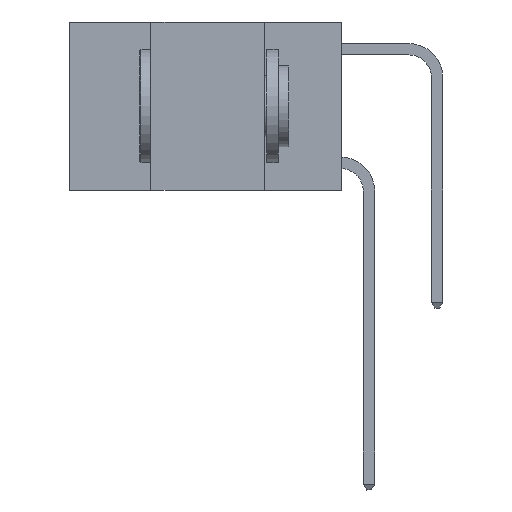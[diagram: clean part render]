
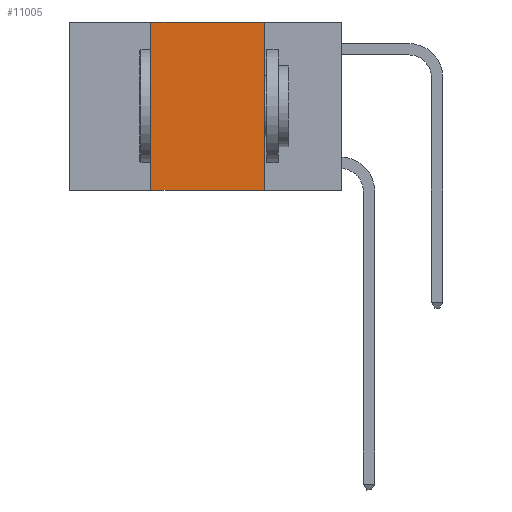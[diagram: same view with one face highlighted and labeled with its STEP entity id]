
A CAD part, left-side view. The second image highlights one B-rep face of the part: STEP entity #11005.
In plain terms, the highlighted planar face has unit normal (-1, 0, 0).
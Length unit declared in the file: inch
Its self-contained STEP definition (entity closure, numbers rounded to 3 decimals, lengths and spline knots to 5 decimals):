
#467 = LINE ( 'NONE', #8551, #8798 ) ;
#986 = DIRECTION ( 'NONE',  ( 0., 0., 1. ) ) ;
#1021 = ORIENTED_EDGE ( 'NONE', *, *, #13815, .F. ) ;
#1459 = EDGE_CURVE ( 'NONE', #10141, #10925, #14796, .T. ) ;
#1756 = DIRECTION ( 'NONE',  ( 0., 0., -1. ) ) ;
#1857 = ORIENTED_EDGE ( 'NONE', *, *, #1459, .T. ) ;
#5733 = CARTESIAN_POINT ( 'NONE',  ( 0., 0.6, 0. ) ) ;
#6305 = AXIS2_PLACEMENT_3D ( 'NONE', #5733, #10704, #1756 ) ;
#6930 = CARTESIAN_POINT ( 'NONE',  ( 0., 0.42, 0. ) ) ;
#7873 = EDGE_CURVE ( 'NONE', #10141, #11492, #16860, .T. ) ;
#8054 = CARTESIAN_POINT ( 'NONE',  ( 0., 0.17, 0. ) ) ;
#8061 = FACE_OUTER_BOUND ( 'NONE', #11272, .T. ) ;
#8293 = DIRECTION ( 'NONE',  ( 0., -1., 0. ) ) ;
#8551 = CARTESIAN_POINT ( 'NONE',  ( 0., 0.6, 0. ) ) ;
#8798 = VECTOR ( 'NONE', #8293, 39.37008 ) ;
#9313 = VECTOR ( 'NONE', #14250, 39.37008 ) ;
#9645 = DIRECTION ( 'NONE',  ( 0., -1., 0. ) ) ;
#10000 = CARTESIAN_POINT ( 'NONE',  ( 0., 0.17, 0. ) ) ;
#10141 = VERTEX_POINT ( 'NONE', #11331 ) ;
#10704 = DIRECTION ( 'NONE',  ( 1., 0., 0. ) ) ;
#10925 = VERTEX_POINT ( 'NONE', #14742 ) ;
#11005 = ADVANCED_FACE ( 'NONE', ( #8061 ), #11993, .F. ) ;
#11272 = EDGE_LOOP ( 'NONE', ( #14204, #1021, #11422, #1857 ) ) ;
#11284 = CARTESIAN_POINT ( 'NONE',  ( 0., 0.42, 0. ) ) ;
#11331 = CARTESIAN_POINT ( 'NONE',  ( 0., 0.42, -0.37 ) ) ;
#11422 = ORIENTED_EDGE ( 'NONE', *, *, #7873, .F. ) ;
#11492 = VERTEX_POINT ( 'NONE', #6930 ) ;
#11591 = LINE ( 'NONE', #10000, #9313 ) ;
#11993 = PLANE ( 'NONE',  #6305 ) ;
#12692 = EDGE_CURVE ( 'NONE', #15018, #10925, #11591, .T. ) ;
#13300 = VECTOR ( 'NONE', #9645, 39.37008 ) ;
#13815 = EDGE_CURVE ( 'NONE', #11492, #15018, #467, .T. ) ;
#14204 = ORIENTED_EDGE ( 'NONE', *, *, #12692, .F. ) ;
#14250 = DIRECTION ( 'NONE',  ( 0., 0., -1. ) ) ;
#14742 = CARTESIAN_POINT ( 'NONE',  ( 0., 0.17, -0.37 ) ) ;
#14796 = LINE ( 'NONE', #16086, #13300 ) ;
#15018 = VERTEX_POINT ( 'NONE', #8054 ) ;
#15544 = VECTOR ( 'NONE', #986, 39.37008 ) ;
#16086 = CARTESIAN_POINT ( 'NONE',  ( 0., 0.6, -0.37 ) ) ;
#16860 = LINE ( 'NONE', #11284, #15544 ) ;
